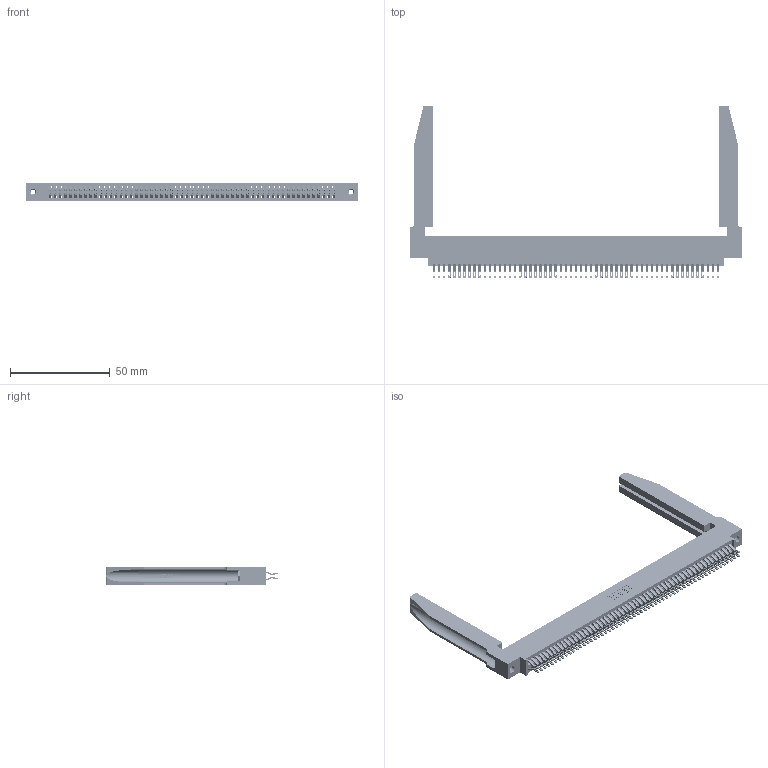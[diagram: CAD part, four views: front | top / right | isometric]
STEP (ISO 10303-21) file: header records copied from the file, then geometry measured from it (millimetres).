
FILE_DESCRIPTION (( 'STEP AP203' ), '1' );
FILE_NAME ('395-114-555-878.STEP', '2019-10-27T18:55:15', ( '' ), ( '' ), 'SwSTEP 2.0', 'SolidWorks 2016', '' );
FILE_SCHEMA (( 'CONFIG_CONTROL_DESIGN' ));
Length unit declared in the file: inch
Products named in the file (5): 345 Part_0.170 Offset - 0.156 Dia-TH; 345-292-001_555 Tail; 345-250-001_345-250-001-102; 345-220-078_345-220-078; 395-114-555-878
Assembly tree (119 placements, depth 2):
  395-114-555-878
    345 Part_0.170 Offset - 0.156 Dia-TH
    345-292-001_555 Tail  x114
    345-250-001_345-250-001-102  x2
    345-220-078_345-220-078  x2
Bounding box: 166.01 x 86.41 x 9.4 mm (x, y, z)
Volume: 24253.8 mm3; surface area: 32787.6 mm2
Topology: 119 solids, 119 shells, 6748 faces, 21139 edges, 14082 vertices
Faces by surface type: plane 3760, cylinder 2936, bspline 36, cone 12, torus 4
Entity records: 47902 total; most frequent: CARTESIAN_POINT 8969, ORIENTED_EDGE 7770, DIRECTION 6851, EDGE_CURVE 3885, VECTOR 3411, LINE 3411, VERTEX_POINT 2584, AXIS2_PLACEMENT_3D 1720
